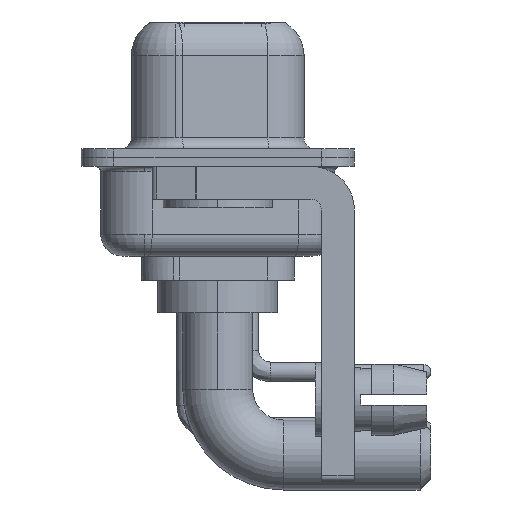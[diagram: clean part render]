
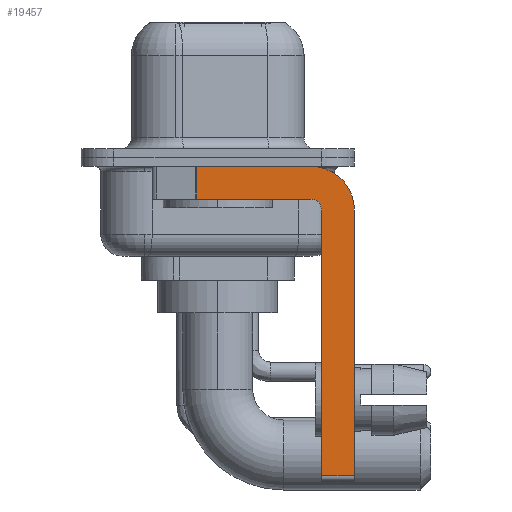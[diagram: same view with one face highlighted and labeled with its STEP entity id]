
A CAD part, left-side view. The second image highlights one B-rep face of the part: STEP entity #19457.
In plain terms, the highlighted planar face has unit normal (-1, 0, 0).
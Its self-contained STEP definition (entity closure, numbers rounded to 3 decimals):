
#390 = CARTESIAN_POINT ( 'NONE',  ( -2.9, -6.25, -14.55 ) ) ;
#647 = DIRECTION ( 'NONE',  ( 0., 0., -1. ) ) ;
#729 = ORIENTED_EDGE ( 'NONE', *, *, #12792, .T. ) ;
#794 = ORIENTED_EDGE ( 'NONE', *, *, #6552, .F. ) ;
#879 = EDGE_CURVE ( 'NONE', #12253, #15447, #10933, .T. ) ;
#1324 = AXIS2_PLACEMENT_3D ( 'NONE', #16160, #2743, #10077 ) ;
#1481 = CARTESIAN_POINT ( 'NONE',  ( -2.9, -4.25, -2.4 ) ) ;
#1921 = DIRECTION ( 'NONE',  ( 0., 0., 1. ) ) ;
#2566 = CARTESIAN_POINT ( 'NONE',  ( -2.9, -4.75, -14.55 ) ) ;
#2740 = CARTESIAN_POINT ( 'NONE',  ( -2.9, -4.75, -2.4 ) ) ;
#2743 = DIRECTION ( 'NONE',  ( 1., 0., 0. ) ) ;
#2771 = DIRECTION ( 'NONE',  ( -1., 0., 0. ) ) ;
#2854 = AXIS2_PLACEMENT_3D ( 'NONE', #10031, #5194, #18813 ) ;
#2998 = EDGE_LOOP ( 'NONE', ( #8405, #6414, #14078, #15657, #794, #729, #10306, #11695 ) ) ;
#3158 = VERTEX_POINT ( 'NONE', #2740 ) ;
#3294 = DIRECTION ( 'NONE',  ( 0., 1., 0. ) ) ;
#3542 = DIRECTION ( 'NONE',  ( 0., -1., 0. ) ) ;
#3761 = CARTESIAN_POINT ( 'NONE',  ( -2.9, -4.25, -1.9 ) ) ;
#3777 = VECTOR ( 'NONE', #1921, 1000. ) ;
#4224 = VERTEX_POINT ( 'NONE', #15770 ) ;
#4238 = VERTEX_POINT ( 'NONE', #9398 ) ;
#4459 = DIRECTION ( 'NONE',  ( 0., 0., 1. ) ) ;
#4892 = DIRECTION ( 'NONE',  ( 0., -1., 0. ) ) ;
#5194 = DIRECTION ( 'NONE',  ( 1., 0., 0. ) ) ;
#5524 = LINE ( 'NONE', #8189, #18473 ) ;
#6010 = VECTOR ( 'NONE', #3542, 1000. ) ;
#6336 = CIRCLE ( 'NONE', #2854, 2. ) ;
#6414 = ORIENTED_EDGE ( 'NONE', *, *, #14960, .T. ) ;
#6552 = EDGE_CURVE ( 'NONE', #13859, #3158, #9454, .T. ) ;
#7005 = FACE_OUTER_BOUND ( 'NONE', #2998, .T. ) ;
#8189 = CARTESIAN_POINT ( 'NONE',  ( -2.9, 0.978, -1.9 ) ) ;
#8266 = CARTESIAN_POINT ( 'NONE',  ( -2.9, -4.25, -0.4 ) ) ;
#8405 = ORIENTED_EDGE ( 'NONE', *, *, #10144, .F. ) ;
#9398 = CARTESIAN_POINT ( 'NONE',  ( -2.9, 0.978, -0.4 ) ) ;
#9454 = LINE ( 'NONE', #18537, #3777 ) ;
#9788 = CARTESIAN_POINT ( 'NONE',  ( -2.9, -4.25, -14.55 ) ) ;
#9854 = CARTESIAN_POINT ( 'NONE',  ( -2.9, 0.978, -1.9 ) ) ;
#10031 = CARTESIAN_POINT ( 'NONE',  ( -2.9, -4.25, -2.4 ) ) ;
#10077 = DIRECTION ( 'NONE',  ( 0., 0., -1. ) ) ;
#10144 = EDGE_CURVE ( 'NONE', #4238, #15517, #17919, .T. ) ;
#10306 = ORIENTED_EDGE ( 'NONE', *, *, #16333, .F. ) ;
#10933 = LINE ( 'NONE', #17201, #11756 ) ;
#11695 = ORIENTED_EDGE ( 'NONE', *, *, #13289, .F. ) ;
#11756 = VECTOR ( 'NONE', #3294, 1000. ) ;
#12253 = VERTEX_POINT ( 'NONE', #3761 ) ;
#12277 = LINE ( 'NONE', #18367, #17511 ) ;
#12307 = VERTEX_POINT ( 'NONE', #390 ) ;
#12792 = EDGE_CURVE ( 'NONE', #13859, #12307, #14075, .T. ) ;
#12966 = DIRECTION ( 'NONE',  ( 0., 0., -1. ) ) ;
#13289 = EDGE_CURVE ( 'NONE', #15517, #4224, #6336, .T. ) ;
#13859 = VERTEX_POINT ( 'NONE', #2566 ) ;
#14075 = LINE ( 'NONE', #9788, #6010 ) ;
#14078 = ORIENTED_EDGE ( 'NONE', *, *, #879, .F. ) ;
#14307 = EDGE_CURVE ( 'NONE', #3158, #12253, #14947, .T. ) ;
#14543 = VECTOR ( 'NONE', #4892, 1000. ) ;
#14947 = CIRCLE ( 'NONE', #16223, 0.5 ) ;
#14960 = EDGE_CURVE ( 'NONE', #4238, #15447, #5524, .T. ) ;
#15447 = VERTEX_POINT ( 'NONE', #9854 ) ;
#15517 = VERTEX_POINT ( 'NONE', #8266 ) ;
#15657 = ORIENTED_EDGE ( 'NONE', *, *, #14307, .F. ) ;
#15770 = CARTESIAN_POINT ( 'NONE',  ( -2.9, -6.25, -2.4 ) ) ;
#16160 = CARTESIAN_POINT ( 'NONE',  ( -2.9, -4.25, -2.4 ) ) ;
#16223 = AXIS2_PLACEMENT_3D ( 'NONE', #1481, #2771, #4459 ) ;
#16333 = EDGE_CURVE ( 'NONE', #4224, #12307, #12277, .T. ) ;
#17201 = CARTESIAN_POINT ( 'NONE',  ( -2.9, -4.25, -1.9 ) ) ;
#17511 = VECTOR ( 'NONE', #12966, 1000. ) ;
#17919 = LINE ( 'NONE', #18515, #14543 ) ;
#18367 = CARTESIAN_POINT ( 'NONE',  ( -2.9, -6.25, -2.4 ) ) ;
#18473 = VECTOR ( 'NONE', #647, 1000. ) ;
#18515 = CARTESIAN_POINT ( 'NONE',  ( -2.9, 3., -0.4 ) ) ;
#18537 = CARTESIAN_POINT ( 'NONE',  ( -2.9, -4.75, -14.8 ) ) ;
#18813 = DIRECTION ( 'NONE',  ( 0., 0., -1. ) ) ;
#19164 = PLANE ( 'NONE',  #1324 ) ;
#19457 = ADVANCED_FACE ( 'NONE', ( #7005 ), #19164, .F. ) ;
